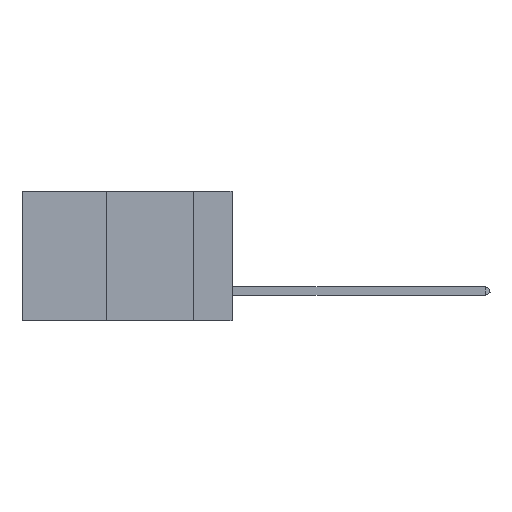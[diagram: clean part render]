
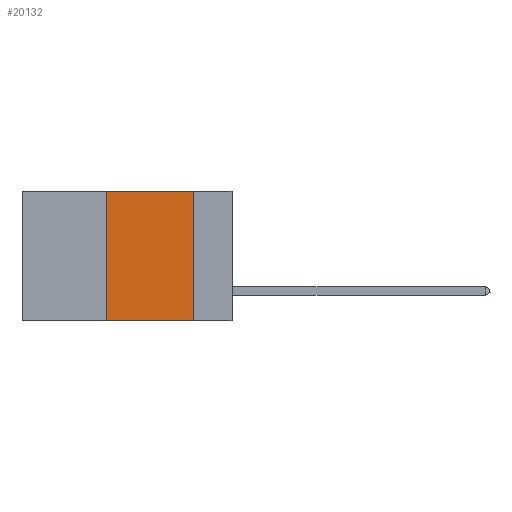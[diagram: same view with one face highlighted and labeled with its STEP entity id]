
A CAD part, left-side view. The second image highlights one B-rep face of the part: STEP entity #20132.
In plain terms, the highlighted planar face has unit normal (-1, 0, 0).
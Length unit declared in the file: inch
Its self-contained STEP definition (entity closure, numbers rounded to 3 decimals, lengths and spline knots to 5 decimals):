
#149 = EDGE_CURVE ( 'NONE', #5824, #20078, #13664, .T. ) ;
#732 = DIRECTION ( 'NONE',  ( 0., 0., -1. ) ) ;
#1777 = EDGE_LOOP ( 'NONE', ( #13493, #18151, #9263, #2649 ) ) ;
#2273 = DIRECTION ( 'NONE',  ( 1., 0., 0. ) ) ;
#2649 = ORIENTED_EDGE ( 'NONE', *, *, #12315, .T. ) ;
#3096 = CARTESIAN_POINT ( 'NONE',  ( 0., 0.36, 0. ) ) ;
#4061 = DIRECTION ( 'NONE',  ( 0., 0., 1. ) ) ;
#4782 = DIRECTION ( 'NONE',  ( 0., -1., 0. ) ) ;
#4905 = DIRECTION ( 'NONE',  ( 0., 0., -1. ) ) ;
#5824 = VERTEX_POINT ( 'NONE', #11263 ) ;
#6899 = VECTOR ( 'NONE', #4782, 39.37008 ) ;
#6919 = VECTOR ( 'NONE', #4061, 39.37008 ) ;
#7036 = FACE_OUTER_BOUND ( 'NONE', #1777, .T. ) ;
#8661 = CARTESIAN_POINT ( 'NONE',  ( 0., 0.6, 0. ) ) ;
#9263 = ORIENTED_EDGE ( 'NONE', *, *, #17135, .F. ) ;
#9375 = CARTESIAN_POINT ( 'NONE',  ( 0., 0.11, -0.37 ) ) ;
#9575 = CARTESIAN_POINT ( 'NONE',  ( 0., 0.36, 0. ) ) ;
#9680 = CARTESIAN_POINT ( 'NONE',  ( 0., 0.11, 0. ) ) ;
#10444 = LINE ( 'NONE', #9575, #6919 ) ;
#10715 = LINE ( 'NONE', #18798, #6899 ) ;
#10962 = PLANE ( 'NONE',  #15306 ) ;
#11263 = CARTESIAN_POINT ( 'NONE',  ( 0., 0.11, 0. ) ) ;
#12315 = EDGE_CURVE ( 'NONE', #21574, #20078, #21072, .T. ) ;
#13493 = ORIENTED_EDGE ( 'NONE', *, *, #149, .F. ) ;
#13664 = LINE ( 'NONE', #9680, #16382 ) ;
#14079 = VERTEX_POINT ( 'NONE', #3096 ) ;
#14080 = VECTOR ( 'NONE', #16076, 39.37008 ) ;
#15306 = AXIS2_PLACEMENT_3D ( 'NONE', #8661, #2273, #732 ) ;
#16076 = DIRECTION ( 'NONE',  ( 0., -1., 0. ) ) ;
#16382 = VECTOR ( 'NONE', #4905, 39.37008 ) ;
#17135 = EDGE_CURVE ( 'NONE', #21574, #14079, #10444, .T. ) ;
#17351 = EDGE_CURVE ( 'NONE', #14079, #5824, #10715, .T. ) ;
#18063 = CARTESIAN_POINT ( 'NONE',  ( 0., 0.36, -0.37 ) ) ;
#18151 = ORIENTED_EDGE ( 'NONE', *, *, #17351, .F. ) ;
#18798 = CARTESIAN_POINT ( 'NONE',  ( 0., 0.6, 0. ) ) ;
#19545 = CARTESIAN_POINT ( 'NONE',  ( 0., 0.6, -0.37 ) ) ;
#20078 = VERTEX_POINT ( 'NONE', #9375 ) ;
#20132 = ADVANCED_FACE ( 'NONE', ( #7036 ), #10962, .F. ) ;
#21072 = LINE ( 'NONE', #19545, #14080 ) ;
#21574 = VERTEX_POINT ( 'NONE', #18063 ) ;
